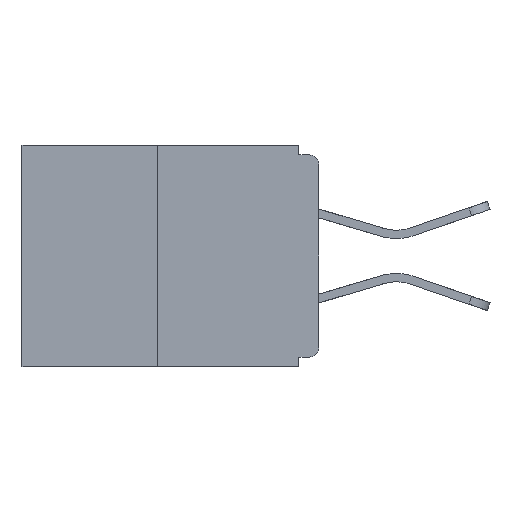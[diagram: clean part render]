
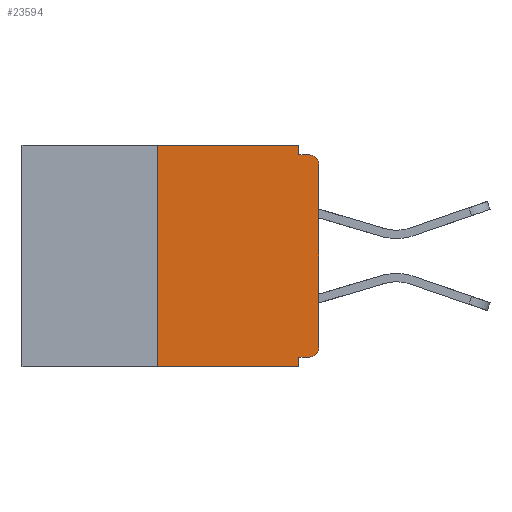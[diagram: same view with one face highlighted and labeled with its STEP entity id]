
A CAD part, left-side view. The second image highlights one B-rep face of the part: STEP entity #23594.
In plain terms, the highlighted planar face has unit normal (-1, 0, 0).
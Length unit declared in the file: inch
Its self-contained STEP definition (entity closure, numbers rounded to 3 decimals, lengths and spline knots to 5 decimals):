
#1185 = CARTESIAN_POINT ( 'NONE',  ( 0., 0.015, -0.03 ) ) ;
#1613 = DIRECTION ( 'NONE',  ( 0., -1., 0. ) ) ;
#2294 = ORIENTED_EDGE ( 'NONE', *, *, #22304, .F. ) ;
#2510 = CARTESIAN_POINT ( 'NONE',  ( 0., 0.015, -0.015 ) ) ;
#3007 = CARTESIAN_POINT ( 'NONE',  ( 0., 0.015, -0.328 ) ) ;
#3064 = CARTESIAN_POINT ( 'NONE',  ( 0., 0.25, 0. ) ) ;
#3446 = DIRECTION ( 'NONE',  ( -1., 0., 0. ) ) ;
#3476 = ORIENTED_EDGE ( 'NONE', *, *, #5969, .F. ) ;
#3646 = ORIENTED_EDGE ( 'NONE', *, *, #20406, .F. ) ;
#4596 = DIRECTION ( 'NONE',  ( 0., 0., -1. ) ) ;
#4672 = VECTOR ( 'NONE', #1613, 39.37008 ) ;
#5452 = CARTESIAN_POINT ( 'NONE',  ( 0., 0.031, -0.015 ) ) ;
#5549 = EDGE_CURVE ( 'NONE', #23230, #25172, #10453, .T. ) ;
#5676 = LINE ( 'NONE', #8129, #14633 ) ;
#5969 = EDGE_CURVE ( 'NONE', #23230, #18249, #27372, .T. ) ;
#6298 = CARTESIAN_POINT ( 'NONE',  ( 0., 0., -0.015 ) ) ;
#6887 = VERTEX_POINT ( 'NONE', #9040 ) ;
#6906 = DIRECTION ( 'NONE',  ( 1., 0., 0. ) ) ;
#7104 = VERTEX_POINT ( 'NONE', #28231 ) ;
#7410 = ORIENTED_EDGE ( 'NONE', *, *, #20414, .F. ) ;
#7438 = EDGE_CURVE ( 'NONE', #24832, #7104, #5676, .T. ) ;
#7947 = AXIS2_PLACEMENT_3D ( 'NONE', #9964, #28488, #19398 ) ;
#8129 = CARTESIAN_POINT ( 'NONE',  ( 0., 0.46, -0.343 ) ) ;
#8174 = CARTESIAN_POINT ( 'NONE',  ( 0., 0.031, 0. ) ) ;
#8971 = VECTOR ( 'NONE', #24357, 39.37008 ) ;
#9040 = CARTESIAN_POINT ( 'NONE',  ( 0., 0.25, 0. ) ) ;
#9045 = DIRECTION ( 'NONE',  ( 0., -1., 0. ) ) ;
#9055 = CARTESIAN_POINT ( 'NONE',  ( 0., 0.46, 0. ) ) ;
#9366 = ORIENTED_EDGE ( 'NONE', *, *, #26594, .T. ) ;
#9472 = CARTESIAN_POINT ( 'NONE',  ( 0., 0., 0. ) ) ;
#9964 = CARTESIAN_POINT ( 'NONE',  ( 0., 0.015, -0.313 ) ) ;
#10138 = VECTOR ( 'NONE', #23545, 39.37008 ) ;
#10453 = CIRCLE ( 'NONE', #7947, 0.015 ) ;
#10603 = ORIENTED_EDGE ( 'NONE', *, *, #28853, .T. ) ;
#11086 = EDGE_CURVE ( 'NONE', #6887, #24090, #18871, .T. ) ;
#11345 = VECTOR ( 'NONE', #15557, 39.37008 ) ;
#11650 = CARTESIAN_POINT ( 'NONE',  ( 0., 0.031, -0.328 ) ) ;
#11810 = DIRECTION ( 'NONE',  ( 0., 0., -1. ) ) ;
#12745 = VERTEX_POINT ( 'NONE', #28270 ) ;
#13968 = LINE ( 'NONE', #9472, #8971 ) ;
#14633 = VECTOR ( 'NONE', #9045, 39.37008 ) ;
#14937 = CIRCLE ( 'NONE', #17162, 0.015 ) ;
#15557 = DIRECTION ( 'NONE',  ( 0., -1., 0. ) ) ;
#16294 = CARTESIAN_POINT ( 'NONE',  ( 0., 0.031, 0. ) ) ;
#16496 = CARTESIAN_POINT ( 'NONE',  ( 0., 0., -0.313 ) ) ;
#17162 = AXIS2_PLACEMENT_3D ( 'NONE', #1185, #3446, #19502 ) ;
#18070 = ORIENTED_EDGE ( 'NONE', *, *, #11086, .F. ) ;
#18120 = CARTESIAN_POINT ( 'NONE',  ( 0., 0.46, 0. ) ) ;
#18249 = VERTEX_POINT ( 'NONE', #11650 ) ;
#18328 = FACE_OUTER_BOUND ( 'NONE', #28683, .T. ) ;
#18871 = LINE ( 'NONE', #9055, #11345 ) ;
#18904 = ORIENTED_EDGE ( 'NONE', *, *, #7438, .T. ) ;
#19070 = DIRECTION ( 'NONE',  ( 0., 1., 0. ) ) ;
#19398 = DIRECTION ( 'NONE',  ( 0., 0., -1. ) ) ;
#19502 = DIRECTION ( 'NONE',  ( 0., 0., -1. ) ) ;
#20406 = EDGE_CURVE ( 'NONE', #18249, #7104, #24269, .T. ) ;
#20414 = EDGE_CURVE ( 'NONE', #24090, #22006, #23539, .T. ) ;
#20430 = VERTEX_POINT ( 'NONE', #2510 ) ;
#20550 = DIRECTION ( 'NONE',  ( 0., 0., -1. ) ) ;
#20645 = PLANE ( 'NONE',  #25457 ) ;
#20954 = CARTESIAN_POINT ( 'NONE',  ( 0., 0.031, -0.343 ) ) ;
#21377 = CARTESIAN_POINT ( 'NONE',  ( 0., 0.25, -0.343 ) ) ;
#21481 = CARTESIAN_POINT ( 'NONE',  ( 0., 0., -0.328 ) ) ;
#21939 = VECTOR ( 'NONE', #19070, 39.37008 ) ;
#22006 = VERTEX_POINT ( 'NONE', #5452 ) ;
#22304 = EDGE_CURVE ( 'NONE', #24832, #6887, #28533, .T. ) ;
#22617 = ORIENTED_EDGE ( 'NONE', *, *, #5549, .T. ) ;
#22988 = LINE ( 'NONE', #6298, #4672 ) ;
#23230 = VERTEX_POINT ( 'NONE', #3007 ) ;
#23539 = LINE ( 'NONE', #16294, #26798 ) ;
#23545 = DIRECTION ( 'NONE',  ( 0., 0., 1. ) ) ;
#23594 = ADVANCED_FACE ( 'NONE', ( #18328 ), #20645, .F. ) ;
#24090 = VERTEX_POINT ( 'NONE', #8174 ) ;
#24269 = LINE ( 'NONE', #20954, #25359 ) ;
#24357 = DIRECTION ( 'NONE',  ( 0., 0., 1. ) ) ;
#24832 = VERTEX_POINT ( 'NONE', #21377 ) ;
#25172 = VERTEX_POINT ( 'NONE', #16496 ) ;
#25359 = VECTOR ( 'NONE', #4596, 39.37008 ) ;
#25457 = AXIS2_PLACEMENT_3D ( 'NONE', #18120, #6906, #20550 ) ;
#26594 = EDGE_CURVE ( 'NONE', #12745, #20430, #14937, .T. ) ;
#26798 = VECTOR ( 'NONE', #11810, 39.37008 ) ;
#27372 = LINE ( 'NONE', #21481, #21939 ) ;
#28231 = CARTESIAN_POINT ( 'NONE',  ( 0., 0.031, -0.343 ) ) ;
#28270 = CARTESIAN_POINT ( 'NONE',  ( 0., 0., -0.03 ) ) ;
#28488 = DIRECTION ( 'NONE',  ( -1., 0., 0. ) ) ;
#28533 = LINE ( 'NONE', #3064, #10138 ) ;
#28545 = EDGE_CURVE ( 'NONE', #22006, #20430, #22988, .T. ) ;
#28683 = EDGE_LOOP ( 'NONE', ( #18070, #2294, #18904, #3646, #3476, #22617, #10603, #9366, #28857, #7410 ) ) ;
#28853 = EDGE_CURVE ( 'NONE', #25172, #12745, #13968, .T. ) ;
#28857 = ORIENTED_EDGE ( 'NONE', *, *, #28545, .F. ) ;
